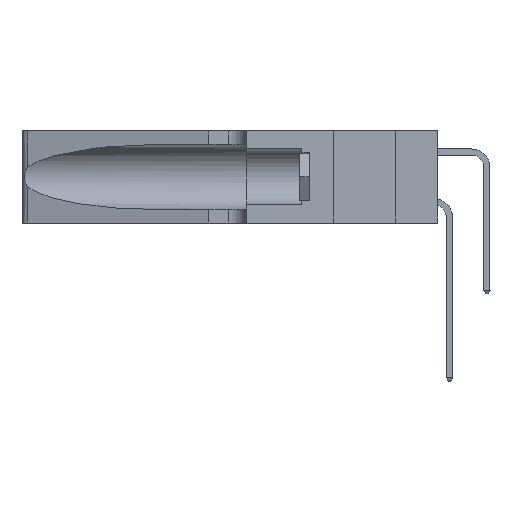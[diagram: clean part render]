
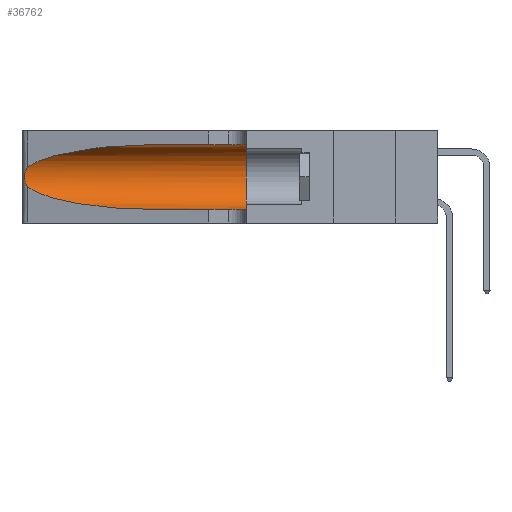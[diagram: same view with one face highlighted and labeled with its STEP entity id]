
A CAD part, left-side view. The second image highlights one B-rep face of the part: STEP entity #36762.
In plain terms, the highlighted cylindrical face has radius 3.308 mm (diameter 6.617 mm), a partial arc.
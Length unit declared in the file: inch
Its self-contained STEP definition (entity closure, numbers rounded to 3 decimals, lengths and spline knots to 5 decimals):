
#22 = EDGE_CURVE ( 'NONE', #35526, #6317, #36020, .T. ) ;
#44 = EDGE_CURVE ( 'NONE', #6857, #44846, #44049, .T. ) ;
#2632 = CARTESIAN_POINT ( 'NONE',  ( 0.1305, 1.61858, 0.05475 ) ) ;
#4753 = CARTESIAN_POINT ( 'NONE',  ( 0.25487, 1.22718, 0.22369 ) ) ;
#4973 = ORIENTED_EDGE ( 'NONE', *, *, #26821, .T. ) ;
#5272 = CARTESIAN_POINT ( 'NONE',  ( 0.26017, 1.23833, 0.17102 ) ) ;
#5808 = CARTESIAN_POINT ( 'NONE',  ( 0.1305, 0.35, 0.185 ) ) ;
#6317 = VERTEX_POINT ( 'NONE', #26052 ) ;
#6857 = VERTEX_POINT ( 'NONE', #12862 ) ;
#8488 = VECTOR ( 'NONE', #24057, 39.37008 ) ;
#8830 = CARTESIAN_POINT ( 'NONE',  ( 0.25787, 1.23484, 0.2124 ) ) ;
#9350 = DIRECTION ( 'NONE',  ( 0., 0., 1. ) ) ;
#12397 = CARTESIAN_POINT ( 'NONE',  ( 0.25856, 1.23593, 0.16098 ) ) ;
#12862 = CARTESIAN_POINT ( 'NONE',  ( 0.1305, 0.72297, 0.31525 ) ) ;
#12923 = CARTESIAN_POINT ( 'NONE',  ( 0.2373, 1.15595, 0.28018 ) ) ;
#13691 = CIRCLE ( 'NONE', #31134, 0.13025 ) ;
#14287 = CARTESIAN_POINT ( 'NONE',  ( 0.25487, 1.22718, 0.14631 ) ) ;
#14422 = CARTESIAN_POINT ( 'NONE',  ( 0.1305, 0.72297, 0.05475 ) ) ;
#14686 = CYLINDRICAL_SURFACE ( 'NONE', #17027, 0.13025 ) ;
#15935 = CARTESIAN_POINT ( 'NONE',  ( 0.25789, 1.23486, 0.15765 ) ) ;
#16456 = DIRECTION ( 'NONE',  ( 0., 1., 0. ) ) ;
#16863 = CARTESIAN_POINT ( 'NONE',  ( 0.25487, 1.22718, 0.14631 ) ) ;
#17027 = AXIS2_PLACEMENT_3D ( 'NONE', #43301, #25207, #28828 ) ;
#19496 = CARTESIAN_POINT ( 'NONE',  ( 0.25555, 1.22993, 0.14849 ) ) ;
#19624 = CARTESIAN_POINT ( 'NONE',  ( 0.1305, 1.61858, 0.31525 ) ) ;
#20936 = ORIENTED_EDGE ( 'NONE', *, *, #28893, .F. ) ;
#22694 = ORIENTED_EDGE ( 'NONE', *, *, #32850, .T. ) ;
#22697 = CARTESIAN_POINT ( 'NONE',  ( 0.25555, 1.22994, 0.2215 ) ) ;
#22852 = CARTESIAN_POINT ( 'NONE',  ( 0.26075, 1.23896, 0.19203 ) ) ;
#23205 = DIRECTION ( 'NONE',  ( 0., -1., 0. ) ) ;
#23713 = CARTESIAN_POINT ( 'NONE',  ( 0.1305, 0.35, 0.31525 ) ) ;
#23860 = CARTESIAN_POINT ( 'NONE',  ( 0.25487, 1.22718, 0.22369 ) ) ;
#24057 = DIRECTION ( 'NONE',  ( 0., -1., 0. ) ) ;
#24134 = FACE_OUTER_BOUND ( 'NONE', #40441, .T. ) ;
#24312 = CARTESIAN_POINT ( 'NONE',  ( 0.1305, 0.72297, 0.05475 ) ) ;
#24582 =( BOUNDED_CURVE ( )  B_SPLINE_CURVE ( 3, ( #14287, #31828, #35694, #14422 ),
 .UNSPECIFIED., .F., .T. ) 
 B_SPLINE_CURVE_WITH_KNOTS ( ( 4, 4 ),
 ( 3.44316, 4.71239 ),
 .UNSPECIFIED. ) 
 CURVE ( )  GEOMETRIC_REPRESENTATION_ITEM ( )  RATIONAL_B_SPLINE_CURVE ( ( 1., 0.87, 0.87, 1. ) ) 
 REPRESENTATION_ITEM ( '' )  );
#25207 = DIRECTION ( 'NONE',  ( 0., -1., 0. ) ) ;
#26052 = CARTESIAN_POINT ( 'NONE',  ( 0.25487, 1.22718, 0.14631 ) ) ;
#26465 = CARTESIAN_POINT ( 'NONE',  ( 0.26075, 1.23896, 0.178 ) ) ;
#26632 = CARTESIAN_POINT ( 'NONE',  ( 0.25487, 1.22718, 0.22369 ) ) ;
#26821 = EDGE_CURVE ( 'NONE', #6857, #35526, #43763, .T. ) ;
#28243 = VERTEX_POINT ( 'NONE', #24312 ) ;
#28828 = DIRECTION ( 'NONE',  ( 0., 0., -1. ) ) ;
#28893 = EDGE_CURVE ( 'NONE', #44846, #39727, #13691, .T. ) ;
#30214 = CARTESIAN_POINT ( 'NONE',  ( 0.26018, 1.23835, 0.19895 ) ) ;
#31134 = AXIS2_PLACEMENT_3D ( 'NONE', #5808, #16456, #9350 ) ;
#31828 = CARTESIAN_POINT ( 'NONE',  ( 0.2373, 1.15595, 0.08982 ) ) ;
#32850 = EDGE_CURVE ( 'NONE', #6317, #28243, #24582, .T. ) ;
#33334 = ORIENTED_EDGE ( 'NONE', *, *, #22, .T. ) ;
#33691 = LINE ( 'NONE', #2632, #39253 ) ;
#35253 = EDGE_CURVE ( 'NONE', #28243, #39727, #33691, .T. ) ;
#35526 = VERTEX_POINT ( 'NONE', #4753 ) ;
#35694 = CARTESIAN_POINT ( 'NONE',  ( 0.18966, 0.96281, 0.05475 ) ) ;
#36013 = ORIENTED_EDGE ( 'NONE', *, *, #44, .F. ) ;
#36020 = B_SPLINE_CURVE_WITH_KNOTS ( 'NONE', 3,
 ( #26632, #22697, #37037, #8830, #44229, #30214, #22852, #26465, #5272, #12397, #15935, #40781, #19496, #16863 ),
 .UNSPECIFIED., .F., .F.,
 ( 4, 2, 2, 2, 2, 2, 4 ),
 ( 0., 0.00027, 0.00053, 0.00107, 0.0016, 0.00187, 0.00214 ),
 .UNSPECIFIED. ) ;
#36762 = ADVANCED_FACE ( 'NONE', ( #24134 ), #14686, .F. ) ;
#37037 = CARTESIAN_POINT ( 'NONE',  ( 0.25639, 1.23184, 0.21858 ) ) ;
#39253 = VECTOR ( 'NONE', #23205, 39.37008 ) ;
#39727 = VERTEX_POINT ( 'NONE', #43191 ) ;
#39940 = ORIENTED_EDGE ( 'NONE', *, *, #35253, .T. ) ;
#40441 = EDGE_LOOP ( 'NONE', ( #4973, #33334, #22694, #39940, #20936, #36013 ) ) ;
#40520 = CARTESIAN_POINT ( 'NONE',  ( 0.18966, 0.96281, 0.31525 ) ) ;
#40781 = CARTESIAN_POINT ( 'NONE',  ( 0.25639, 1.23186, 0.15144 ) ) ;
#43191 = CARTESIAN_POINT ( 'NONE',  ( 0.1305, 0.35, 0.05475 ) ) ;
#43301 = CARTESIAN_POINT ( 'NONE',  ( 0.1305, 1.61858, 0.185 ) ) ;
#43763 =( BOUNDED_CURVE ( )  B_SPLINE_CURVE ( 3, ( #44458, #40520, #12923, #23860 ),
 .UNSPECIFIED., .F., .F. ) 
 B_SPLINE_CURVE_WITH_KNOTS ( ( 4, 4 ),
 ( 1.5708, 2.84003 ),
 .UNSPECIFIED. ) 
 CURVE ( )  GEOMETRIC_REPRESENTATION_ITEM ( )  RATIONAL_B_SPLINE_CURVE ( ( 1., 0.87, 0.87, 1. ) ) 
 REPRESENTATION_ITEM ( '' )  );
#44049 = LINE ( 'NONE', #19624, #8488 ) ;
#44229 = CARTESIAN_POINT ( 'NONE',  ( 0.25854, 1.2359, 0.20912 ) ) ;
#44458 = CARTESIAN_POINT ( 'NONE',  ( 0.1305, 0.72297, 0.31525 ) ) ;
#44846 = VERTEX_POINT ( 'NONE', #23713 ) ;
